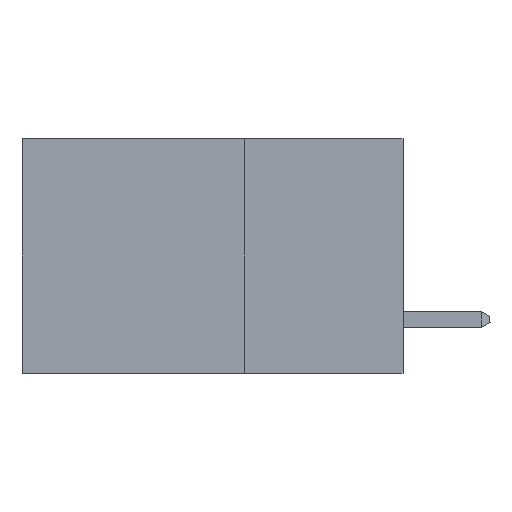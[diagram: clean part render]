
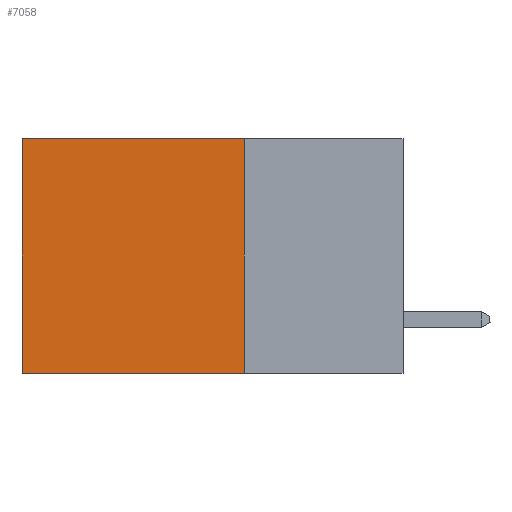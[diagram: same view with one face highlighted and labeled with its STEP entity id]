
A CAD part, left-side view. The second image highlights one B-rep face of the part: STEP entity #7058.
In plain terms, the highlighted planar face has unit normal (-1, 0, 0).
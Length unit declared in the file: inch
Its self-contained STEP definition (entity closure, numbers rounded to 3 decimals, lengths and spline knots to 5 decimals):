
#2402 = EDGE_LOOP ( 'NONE', ( #5380, #19413, #34742, #18332 ) ) ;
#2633 = CARTESIAN_POINT ( 'NONE',  ( 0.2875, 0.6, 0. ) ) ;
#2872 = DIRECTION ( 'NONE',  ( 0., 1., 0. ) ) ;
#5380 = ORIENTED_EDGE ( 'NONE', *, *, #29712, .T. ) ;
#6524 = EDGE_CURVE ( 'NONE', #8829, #33889, #29136, .T. ) ;
#7058 = ADVANCED_FACE ( 'NONE', ( #26322 ), #7135, .F. ) ;
#7135 = PLANE ( 'NONE',  #19266 ) ;
#7519 = LINE ( 'NONE', #10552, #14374 ) ;
#8045 = VECTOR ( 'NONE', #36588, 39.37008 ) ;
#8061 = EDGE_CURVE ( 'NONE', #8829, #36804, #7519, .T. ) ;
#8829 = VERTEX_POINT ( 'NONE', #33005 ) ;
#10396 = LINE ( 'NONE', #2633, #26857 ) ;
#10552 = CARTESIAN_POINT ( 'NONE',  ( 0.2875, 0.25, 0. ) ) ;
#12579 = LINE ( 'NONE', #19119, #8045 ) ;
#12785 = CARTESIAN_POINT ( 'NONE',  ( 0.2875, 0.25, -0.37 ) ) ;
#12882 = EDGE_CURVE ( 'NONE', #36804, #26646, #12579, .T. ) ;
#13005 = DIRECTION ( 'NONE',  ( 0., 0., -1. ) ) ;
#14374 = VECTOR ( 'NONE', #34177, 39.37008 ) ;
#18332 = ORIENTED_EDGE ( 'NONE', *, *, #6524, .T. ) ;
#19119 = CARTESIAN_POINT ( 'NONE',  ( 0.2875, 0.25, -0.37 ) ) ;
#19266 = AXIS2_PLACEMENT_3D ( 'NONE', #30396, #30529, #13005 ) ;
#19413 = ORIENTED_EDGE ( 'NONE', *, *, #12882, .F. ) ;
#20226 = CARTESIAN_POINT ( 'NONE',  ( 0.2875, 0.25, 0. ) ) ;
#22644 = CARTESIAN_POINT ( 'NONE',  ( 0.2875, 0.6, 0. ) ) ;
#25589 = DIRECTION ( 'NONE',  ( 0., 0., -1. ) ) ;
#26322 = FACE_OUTER_BOUND ( 'NONE', #2402, .T. ) ;
#26646 = VERTEX_POINT ( 'NONE', #31923 ) ;
#26857 = VECTOR ( 'NONE', #25589, 39.37008 ) ;
#27775 = VECTOR ( 'NONE', #2872, 39.37008 ) ;
#29136 = LINE ( 'NONE', #20226, #27775 ) ;
#29712 = EDGE_CURVE ( 'NONE', #33889, #26646, #10396, .T. ) ;
#30396 = CARTESIAN_POINT ( 'NONE',  ( 0.2875, 0.25, 0. ) ) ;
#30529 = DIRECTION ( 'NONE',  ( 1., 0., 0. ) ) ;
#31923 = CARTESIAN_POINT ( 'NONE',  ( 0.2875, 0.6, -0.37 ) ) ;
#33005 = CARTESIAN_POINT ( 'NONE',  ( 0.2875, 0.25, 0. ) ) ;
#33889 = VERTEX_POINT ( 'NONE', #22644 ) ;
#34177 = DIRECTION ( 'NONE',  ( 0., 0., -1. ) ) ;
#34742 = ORIENTED_EDGE ( 'NONE', *, *, #8061, .F. ) ;
#36588 = DIRECTION ( 'NONE',  ( 0., 1., 0. ) ) ;
#36804 = VERTEX_POINT ( 'NONE', #12785 ) ;
